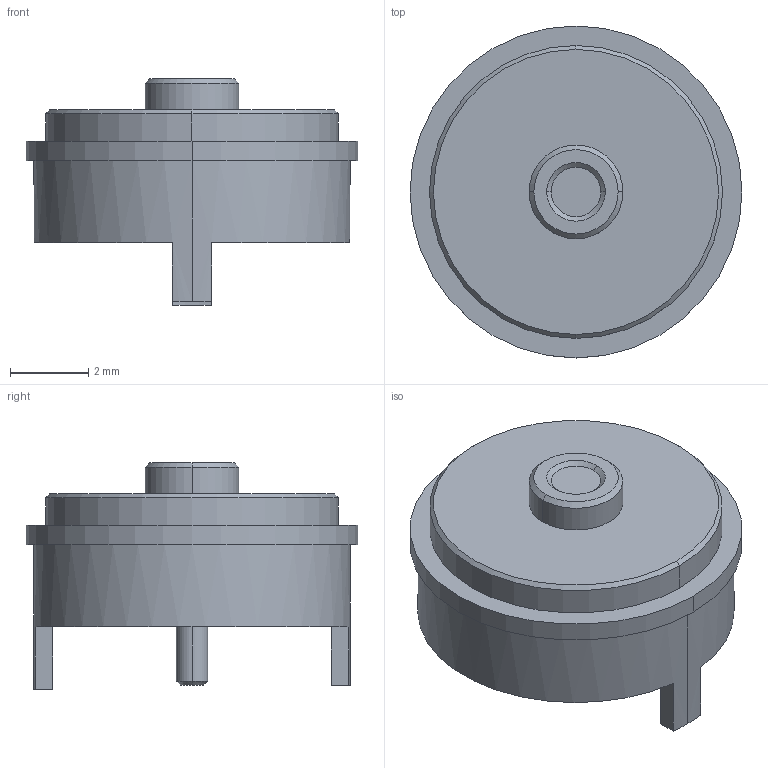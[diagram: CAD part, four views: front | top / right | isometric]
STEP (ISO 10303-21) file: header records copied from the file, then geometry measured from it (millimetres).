
FILE_DESCRIPTION (( 'STEP AP214' ), '1' );
FILE_NAME ('686C02222030C1E.STEP', '2023-04-27T17:39:57', ( '' ), ( '' ), 'SwSTEP 2.0', 'SolidWorks 2020', '' );
FILE_SCHEMA (( 'AUTOMOTIVE_DESIGN' ));
Length unit declared in the file: millimetre
Products named in the file (1): 686C02222030C1E
Bounding box: 8.5 x 8.5 x 5.8 mm (x, y, z)
Volume: 173.9 mm3; surface area: 222.8 mm2
Topology: 2 solids, 2 shells, 43 faces, 90 edges, 58 vertices
Faces by surface type: cylinder 18, plane 17, cone 8
Entity records: 1682 total; most frequent: DIRECTION 228, CARTESIAN_POINT 192, ORIENTED_EDGE 180, AXIS2_PLACEMENT_3D 94, EDGE_CURVE 90, VERTEX_POINT 58, CIRCLE 50, EDGE_LOOP 50
